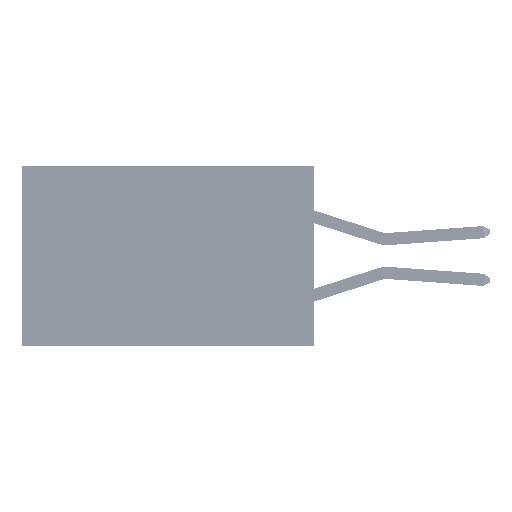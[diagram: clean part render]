
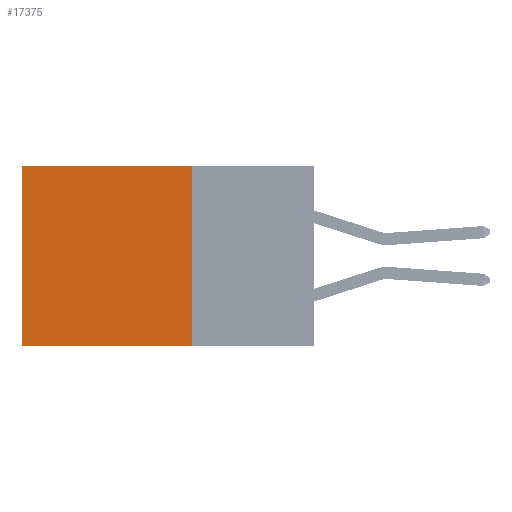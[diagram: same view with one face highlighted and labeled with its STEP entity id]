
A CAD part, left-side view. The second image highlights one B-rep face of the part: STEP entity #17375.
In plain terms, the highlighted planar face has unit normal (-1, 0, 0).
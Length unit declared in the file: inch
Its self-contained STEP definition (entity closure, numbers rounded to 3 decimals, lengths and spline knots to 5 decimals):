
#1116 = DIRECTION ( 'NONE',  ( 0., 0., -1. ) ) ;
#1535 = CARTESIAN_POINT ( 'NONE',  ( 0.2875, 0.25, -0.37 ) ) ;
#2079 = ORIENTED_EDGE ( 'NONE', *, *, #36716, .F. ) ;
#3135 = CARTESIAN_POINT ( 'NONE',  ( 0.2875, 0.6, 0. ) ) ;
#5951 = ORIENTED_EDGE ( 'NONE', *, *, #45042, .F. ) ;
#6317 = CARTESIAN_POINT ( 'NONE',  ( 0.2875, 0.25, 0. ) ) ;
#7396 = DIRECTION ( 'NONE',  ( 0., 0., -1. ) ) ;
#9135 = CARTESIAN_POINT ( 'NONE',  ( 0.2875, 0.25, 0. ) ) ;
#12960 = EDGE_CURVE ( 'NONE', #46133, #25914, #46618, .T. ) ;
#16429 = DIRECTION ( 'NONE',  ( 0., 0., -1. ) ) ;
#17011 = VERTEX_POINT ( 'NONE', #1535 ) ;
#17375 = ADVANCED_FACE ( 'NONE', ( #18602 ), #43627, .F. ) ;
#18602 = FACE_OUTER_BOUND ( 'NONE', #48608, .T. ) ;
#19333 = DIRECTION ( 'NONE',  ( 0., 1., 0. ) ) ;
#20497 = LINE ( 'NONE', #9135, #46806 ) ;
#20819 = LINE ( 'NONE', #48047, #48949 ) ;
#23580 = CARTESIAN_POINT ( 'NONE',  ( 0.2875, 0.25, 0. ) ) ;
#25914 = VERTEX_POINT ( 'NONE', #31035 ) ;
#30638 = EDGE_CURVE ( 'NONE', #25914, #41855, #37629, .T. ) ;
#30904 = VECTOR ( 'NONE', #7396, 39.37008 ) ;
#31035 = CARTESIAN_POINT ( 'NONE',  ( 0.2875, 0.6, 0. ) ) ;
#31751 = AXIS2_PLACEMENT_3D ( 'NONE', #47681, #39821, #16429 ) ;
#36209 = VECTOR ( 'NONE', #19333, 39.37008 ) ;
#36716 = EDGE_CURVE ( 'NONE', #17011, #41855, #20819, .T. ) ;
#37151 = ORIENTED_EDGE ( 'NONE', *, *, #12960, .T. ) ;
#37629 = LINE ( 'NONE', #3135, #30904 ) ;
#39821 = DIRECTION ( 'NONE',  ( 1., 0., 0. ) ) ;
#40029 = DIRECTION ( 'NONE',  ( 0., 1., 0. ) ) ;
#40275 = ORIENTED_EDGE ( 'NONE', *, *, #30638, .T. ) ;
#41855 = VERTEX_POINT ( 'NONE', #47859 ) ;
#43627 = PLANE ( 'NONE',  #31751 ) ;
#45042 = EDGE_CURVE ( 'NONE', #46133, #17011, #20497, .T. ) ;
#46133 = VERTEX_POINT ( 'NONE', #6317 ) ;
#46618 = LINE ( 'NONE', #23580, #36209 ) ;
#46806 = VECTOR ( 'NONE', #1116, 39.37008 ) ;
#47681 = CARTESIAN_POINT ( 'NONE',  ( 0.2875, 0.25, 0. ) ) ;
#47859 = CARTESIAN_POINT ( 'NONE',  ( 0.2875, 0.6, -0.37 ) ) ;
#48047 = CARTESIAN_POINT ( 'NONE',  ( 0.2875, 0.25, -0.37 ) ) ;
#48608 = EDGE_LOOP ( 'NONE', ( #40275, #2079, #5951, #37151 ) ) ;
#48949 = VECTOR ( 'NONE', #40029, 39.37008 ) ;
